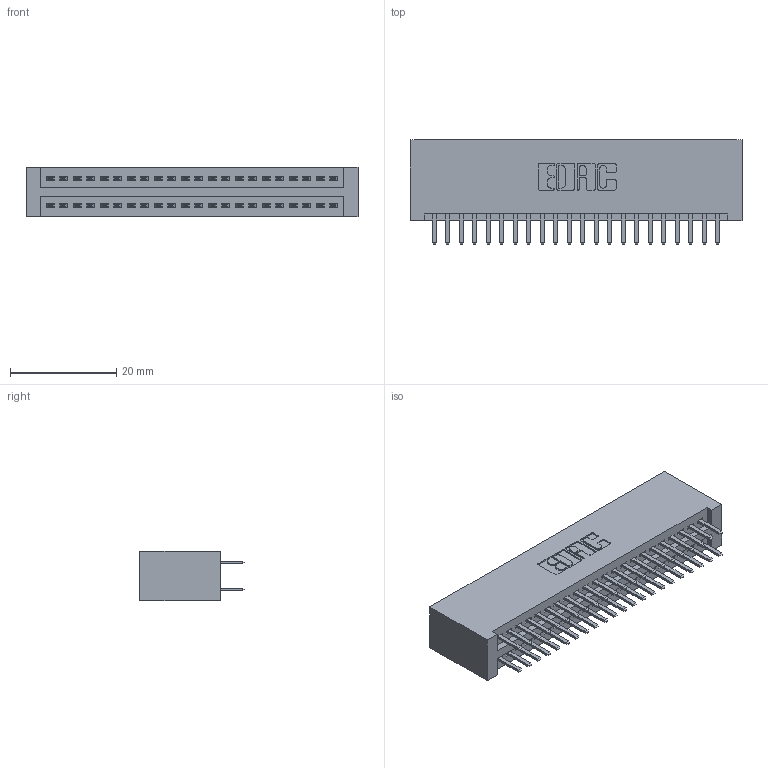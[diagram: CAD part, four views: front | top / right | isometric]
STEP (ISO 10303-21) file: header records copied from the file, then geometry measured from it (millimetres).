
FILE_DESCRIPTION (( 'STEP AP203' ), '1' );
FILE_NAME ('345-044-520-201.STEP', '2018-09-08T08:53:34', ( '' ), ( '' ), 'SwSTEP 2.0', 'SolidWorks 2016', '' );
FILE_SCHEMA (( 'CONFIG_CONTROL_DESIGN' ));
Length unit declared in the file: inch
Products named in the file (3): 345 Part_No Mounting Lugs; 345-292-001_345-293-120; 345-044-520-201
Assembly tree (45 placements, depth 2):
  345-044-520-201
    345 Part_No Mounting Lugs
    345-292-001_345-293-120  x44
Bounding box: 62.48 x 19.68 x 9.4 mm (x, y, z)
Volume: 6480.7 mm3; surface area: 9454.3 mm2
Topology: 45 solids, 45 shells, 2494 faces, 7225 edges, 4698 vertices
Faces by surface type: plane 1616, cylinder 878
Entity records: 19791 total; most frequent: CARTESIAN_POINT 3348, ORIENTED_EDGE 3270, DIRECTION 2959, EDGE_CURVE 1635, VECTOR 1419, LINE 1419, VERTEX_POINT 1086, AXIS2_PLACEMENT_3D 770
